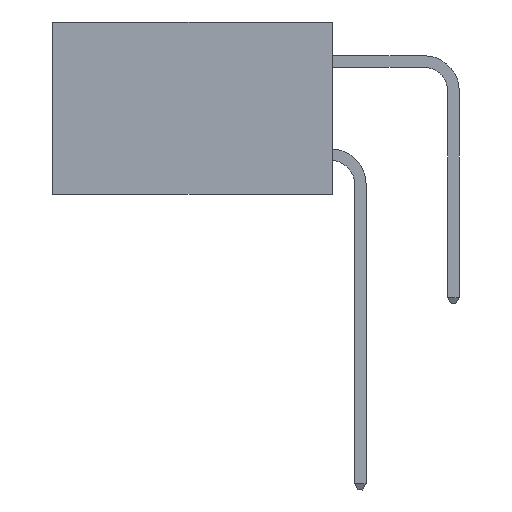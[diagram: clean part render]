
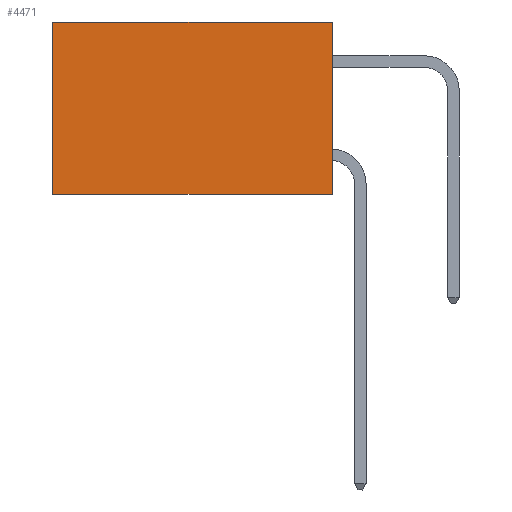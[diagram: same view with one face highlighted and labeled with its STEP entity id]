
A CAD part, left-side view. The second image highlights one B-rep face of the part: STEP entity #4471.
In plain terms, the highlighted planar face has unit normal (-1, 0, 0).
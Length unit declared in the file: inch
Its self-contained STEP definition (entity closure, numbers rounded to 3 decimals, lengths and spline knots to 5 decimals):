
#141 = LINE ( 'NONE', #4248, #11742 ) ;
#181 = ORIENTED_EDGE ( 'NONE', *, *, #13248, .F. ) ;
#677 = VERTEX_POINT ( 'NONE', #5427 ) ;
#961 = DIRECTION ( 'NONE',  ( 1., 0., 0. ) ) ;
#967 = DIRECTION ( 'NONE',  ( 0., 0., -1. ) ) ;
#3250 = LINE ( 'NONE', #13856, #6251 ) ;
#4248 = CARTESIAN_POINT ( 'NONE',  ( 0.298, 0., 0. ) ) ;
#4471 = ADVANCED_FACE ( 'NONE', ( #18308 ), #8859, .F. ) ;
#4606 = VECTOR ( 'NONE', #9195, 39.37008 ) ;
#5102 = ORIENTED_EDGE ( 'NONE', *, *, #13560, .F. ) ;
#5427 = CARTESIAN_POINT ( 'NONE',  ( 0.298, 0., 0. ) ) ;
#6251 = VECTOR ( 'NONE', #15285, 39.37008 ) ;
#8204 = EDGE_LOOP ( 'NONE', ( #18056, #5102, #181, #9911 ) ) ;
#8636 = CARTESIAN_POINT ( 'NONE',  ( 0.298, 0., -0.37 ) ) ;
#8859 = PLANE ( 'NONE',  #9129 ) ;
#9129 = AXIS2_PLACEMENT_3D ( 'NONE', #14083, #961, #967 ) ;
#9188 = VERTEX_POINT ( 'NONE', #8636 ) ;
#9195 = DIRECTION ( 'NONE',  ( 0., 1., 0. ) ) ;
#9315 = CARTESIAN_POINT ( 'NONE',  ( 0.298, 0.6, 0. ) ) ;
#9657 = VECTOR ( 'NONE', #15453, 39.37008 ) ;
#9911 = ORIENTED_EDGE ( 'NONE', *, *, #17342, .T. ) ;
#11742 = VECTOR ( 'NONE', #15731, 39.37008 ) ;
#12250 = LINE ( 'NONE', #17724, #4606 ) ;
#12656 = CARTESIAN_POINT ( 'NONE',  ( 0.298, 0., -0.37 ) ) ;
#13248 = EDGE_CURVE ( 'NONE', #677, #9188, #141, .T. ) ;
#13494 = LINE ( 'NONE', #12656, #9657 ) ;
#13560 = EDGE_CURVE ( 'NONE', #9188, #16270, #13494, .T. ) ;
#13856 = CARTESIAN_POINT ( 'NONE',  ( 0.298, 0.6, 0. ) ) ;
#14083 = CARTESIAN_POINT ( 'NONE',  ( 0.298, 0., 0. ) ) ;
#14688 = VERTEX_POINT ( 'NONE', #9315 ) ;
#15285 = DIRECTION ( 'NONE',  ( 0., 0., -1. ) ) ;
#15453 = DIRECTION ( 'NONE',  ( 0., 1., 0. ) ) ;
#15731 = DIRECTION ( 'NONE',  ( 0., 0., -1. ) ) ;
#16146 = EDGE_CURVE ( 'NONE', #14688, #16270, #3250, .T. ) ;
#16270 = VERTEX_POINT ( 'NONE', #18265 ) ;
#17342 = EDGE_CURVE ( 'NONE', #677, #14688, #12250, .T. ) ;
#17724 = CARTESIAN_POINT ( 'NONE',  ( 0.298, 0., 0. ) ) ;
#18056 = ORIENTED_EDGE ( 'NONE', *, *, #16146, .T. ) ;
#18265 = CARTESIAN_POINT ( 'NONE',  ( 0.298, 0.6, -0.37 ) ) ;
#18308 = FACE_OUTER_BOUND ( 'NONE', #8204, .T. ) ;
